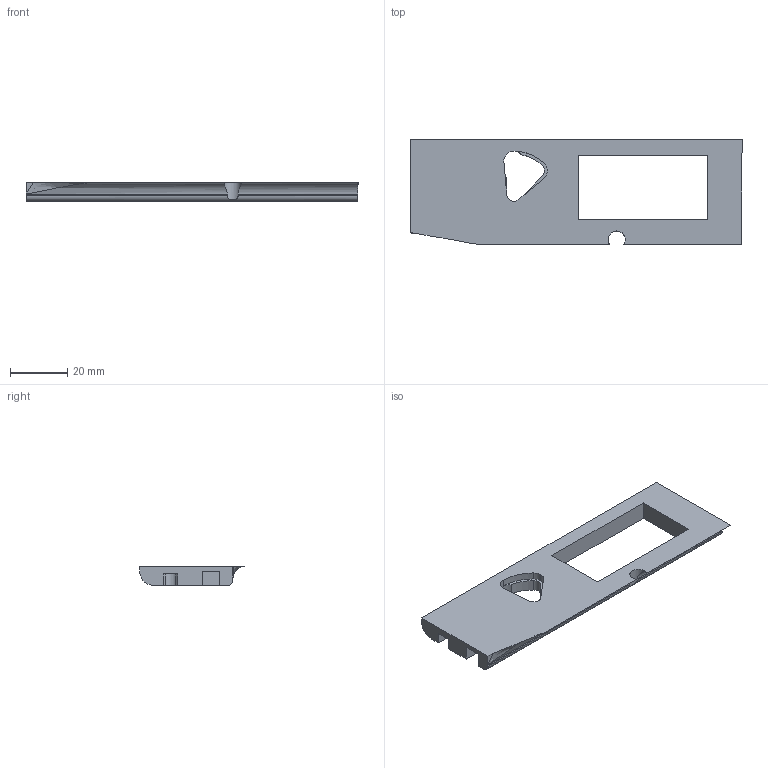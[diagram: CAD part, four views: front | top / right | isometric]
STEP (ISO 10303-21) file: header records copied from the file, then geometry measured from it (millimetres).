
FILE_DESCRIPTION (( 'STEP AP214' ), '1' );
FILE_NAME ('Receiver_Forward_Panel_Left_2.step', '2014-05-14T06:10:09', ( 'WarFairy' ), ( '' ), 'SwSTEP 2.0', 'SolidWorks 2013', '' );
FILE_SCHEMA (( 'AUTOMOTIVE_DESIGN' ));
Length unit declared in the file: inch
Products named in the file (1): Receiver_Forward_Panel_Left_2
Bounding box: 115.7 x 36.5 x 6.57 mm (x, y, z)
Volume: 13952.8 mm3; surface area: 9576.4 mm2
Topology: 1 solids, 1 shells, 54 faces, 143 edges, 93 vertices
Faces by surface type: plane 28, cylinder 25, bspline 1
Entity records: 1949 total; most frequent: CARTESIAN_POINT 542, DIRECTION 286, ORIENTED_EDGE 284, EDGE_CURVE 142, AXIS2_PLACEMENT_3D 99, VERTEX_POINT 93, VECTOR 88, LINE 88
